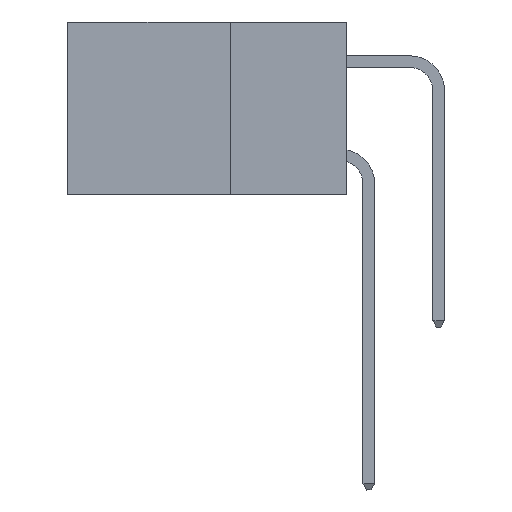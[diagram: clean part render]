
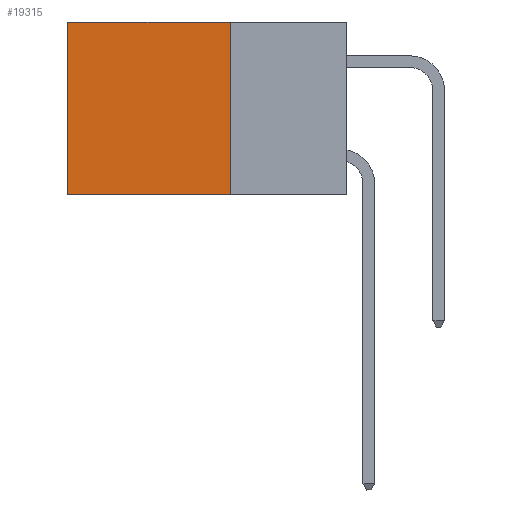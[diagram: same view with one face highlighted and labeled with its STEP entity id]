
A CAD part, left-side view. The second image highlights one B-rep face of the part: STEP entity #19315.
In plain terms, the highlighted planar face has unit normal (-1, 0, 0).
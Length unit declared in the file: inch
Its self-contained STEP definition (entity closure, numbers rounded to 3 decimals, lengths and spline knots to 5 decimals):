
#120 = ORIENTED_EDGE ( 'NONE', *, *, #4264, .F. ) ;
#1557 = VERTEX_POINT ( 'NONE', #10049 ) ;
#1789 = VECTOR ( 'NONE', #14795, 39.37008 ) ;
#1950 = LINE ( 'NONE', #24733, #34305 ) ;
#3604 = CARTESIAN_POINT ( 'NONE',  ( 0.2875, 0.25, 0. ) ) ;
#4264 = EDGE_CURVE ( 'NONE', #26684, #26963, #31005, .T. ) ;
#6168 = LINE ( 'NONE', #3604, #1789 ) ;
#7999 = CARTESIAN_POINT ( 'NONE',  ( 0.2875, 0.6, 0. ) ) ;
#9213 = DIRECTION ( 'NONE',  ( 1., 0., 0. ) ) ;
#10049 = CARTESIAN_POINT ( 'NONE',  ( 0.2875, 0.25, 0. ) ) ;
#11413 = CARTESIAN_POINT ( 'NONE',  ( 0.2875, 0.25, 0. ) ) ;
#11480 = CARTESIAN_POINT ( 'NONE',  ( 0.2875, 0.25, -0.37 ) ) ;
#11631 = VECTOR ( 'NONE', #19210, 39.37008 ) ;
#11904 = EDGE_LOOP ( 'NONE', ( #30135, #120, #35135, #21958 ) ) ;
#14222 = LINE ( 'NONE', #7999, #11631 ) ;
#14380 = EDGE_CURVE ( 'NONE', #1557, #19298, #1950, .T. ) ;
#14795 = DIRECTION ( 'NONE',  ( 0., 0., -1. ) ) ;
#17481 = PLANE ( 'NONE',  #33316 ) ;
#19210 = DIRECTION ( 'NONE',  ( 0., 0., -1. ) ) ;
#19298 = VERTEX_POINT ( 'NONE', #28508 ) ;
#19315 = ADVANCED_FACE ( 'NONE', ( #28160 ), #17481, .F. ) ;
#21958 = ORIENTED_EDGE ( 'NONE', *, *, #14380, .T. ) ;
#22660 = EDGE_CURVE ( 'NONE', #1557, #26684, #6168, .T. ) ;
#22702 = DIRECTION ( 'NONE',  ( 0., 1., 0. ) ) ;
#24195 = DIRECTION ( 'NONE',  ( 0., 1., 0. ) ) ;
#24733 = CARTESIAN_POINT ( 'NONE',  ( 0.2875, 0.25, 0. ) ) ;
#25125 = CARTESIAN_POINT ( 'NONE',  ( 0.2875, 0.25, -0.37 ) ) ;
#26684 = VERTEX_POINT ( 'NONE', #25125 ) ;
#26963 = VERTEX_POINT ( 'NONE', #30398 ) ;
#27660 = VECTOR ( 'NONE', #22702, 39.37008 ) ;
#28160 = FACE_OUTER_BOUND ( 'NONE', #11904, .T. ) ;
#28443 = EDGE_CURVE ( 'NONE', #19298, #26963, #14222, .T. ) ;
#28508 = CARTESIAN_POINT ( 'NONE',  ( 0.2875, 0.6, 0. ) ) ;
#30135 = ORIENTED_EDGE ( 'NONE', *, *, #28443, .T. ) ;
#30398 = CARTESIAN_POINT ( 'NONE',  ( 0.2875, 0.6, -0.37 ) ) ;
#31005 = LINE ( 'NONE', #11480, #27660 ) ;
#33316 = AXIS2_PLACEMENT_3D ( 'NONE', #11413, #9213, #34051 ) ;
#34051 = DIRECTION ( 'NONE',  ( 0., 0., -1. ) ) ;
#34305 = VECTOR ( 'NONE', #24195, 39.37008 ) ;
#35135 = ORIENTED_EDGE ( 'NONE', *, *, #22660, .F. ) ;
